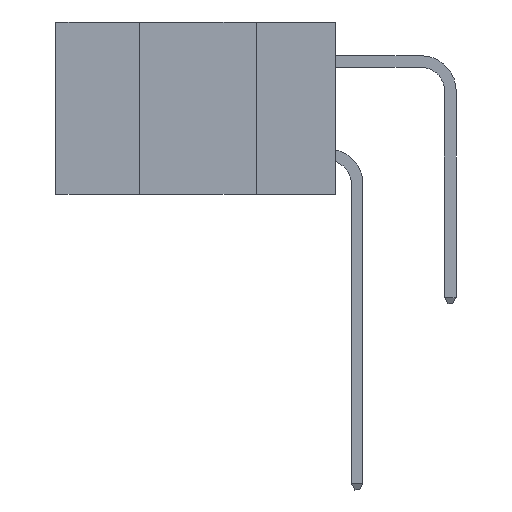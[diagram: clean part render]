
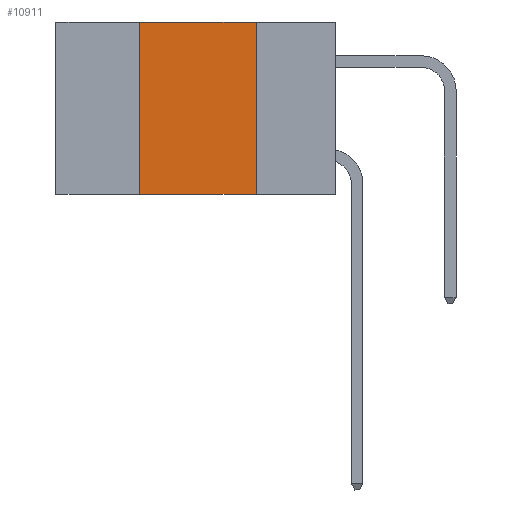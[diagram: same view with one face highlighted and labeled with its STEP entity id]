
A CAD part, left-side view. The second image highlights one B-rep face of the part: STEP entity #10911.
In plain terms, the highlighted planar face has unit normal (-1, 0, 0).
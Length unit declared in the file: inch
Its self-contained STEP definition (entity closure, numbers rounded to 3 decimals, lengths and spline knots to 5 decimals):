
#108 = VERTEX_POINT ( 'NONE', #4191 ) ;
#856 = VERTEX_POINT ( 'NONE', #7234 ) ;
#1320 = DIRECTION ( 'NONE',  ( 0., 0., 1. ) ) ;
#1611 = CARTESIAN_POINT ( 'NONE',  ( 0., 0.42, 0. ) ) ;
#1967 = EDGE_CURVE ( 'NONE', #10652, #10966, #2590, .T. ) ;
#2057 = VECTOR ( 'NONE', #6824, 39.37008 ) ;
#2129 = DIRECTION ( 'NONE',  ( 1., 0., 0. ) ) ;
#2590 = LINE ( 'NONE', #8170, #8199 ) ;
#3165 = FACE_OUTER_BOUND ( 'NONE', #8617, .T. ) ;
#3171 = VECTOR ( 'NONE', #1320, 39.37008 ) ;
#3318 = DIRECTION ( 'NONE',  ( 0., -1., 0. ) ) ;
#4191 = CARTESIAN_POINT ( 'NONE',  ( 0., 0.42, -0.37 ) ) ;
#4479 = ORIENTED_EDGE ( 'NONE', *, *, #1967, .F. ) ;
#4678 = LINE ( 'NONE', #13516, #2057 ) ;
#5489 = EDGE_CURVE ( 'NONE', #108, #10652, #9164, .T. ) ;
#6824 = DIRECTION ( 'NONE',  ( 0., -1., 0. ) ) ;
#6999 = CARTESIAN_POINT ( 'NONE',  ( 0., 0.42, 0. ) ) ;
#7048 = VECTOR ( 'NONE', #11359, 39.37008 ) ;
#7234 = CARTESIAN_POINT ( 'NONE',  ( 0., 0.17, -0.37 ) ) ;
#8170 = CARTESIAN_POINT ( 'NONE',  ( 0., 0.6, 0. ) ) ;
#8199 = VECTOR ( 'NONE', #3318, 39.37008 ) ;
#8617 = EDGE_LOOP ( 'NONE', ( #9554, #4479, #13385, #11132 ) ) ;
#8868 = CARTESIAN_POINT ( 'NONE',  ( 0., 0.6, 0. ) ) ;
#9020 = AXIS2_PLACEMENT_3D ( 'NONE', #8868, #2129, #10035 ) ;
#9164 = LINE ( 'NONE', #6999, #3171 ) ;
#9554 = ORIENTED_EDGE ( 'NONE', *, *, #11077, .F. ) ;
#10035 = DIRECTION ( 'NONE',  ( 0., 0., -1. ) ) ;
#10061 = LINE ( 'NONE', #10219, #7048 ) ;
#10219 = CARTESIAN_POINT ( 'NONE',  ( 0., 0.17, 0. ) ) ;
#10652 = VERTEX_POINT ( 'NONE', #1611 ) ;
#10911 = ADVANCED_FACE ( 'NONE', ( #3165 ), #14389, .F. ) ;
#10966 = VERTEX_POINT ( 'NONE', #14439 ) ;
#11077 = EDGE_CURVE ( 'NONE', #10966, #856, #10061, .T. ) ;
#11132 = ORIENTED_EDGE ( 'NONE', *, *, #12828, .T. ) ;
#11359 = DIRECTION ( 'NONE',  ( 0., 0., -1. ) ) ;
#12828 = EDGE_CURVE ( 'NONE', #108, #856, #4678, .T. ) ;
#13385 = ORIENTED_EDGE ( 'NONE', *, *, #5489, .F. ) ;
#13516 = CARTESIAN_POINT ( 'NONE',  ( 0., 0.6, -0.37 ) ) ;
#14389 = PLANE ( 'NONE',  #9020 ) ;
#14439 = CARTESIAN_POINT ( 'NONE',  ( 0., 0.17, 0. ) ) ;
